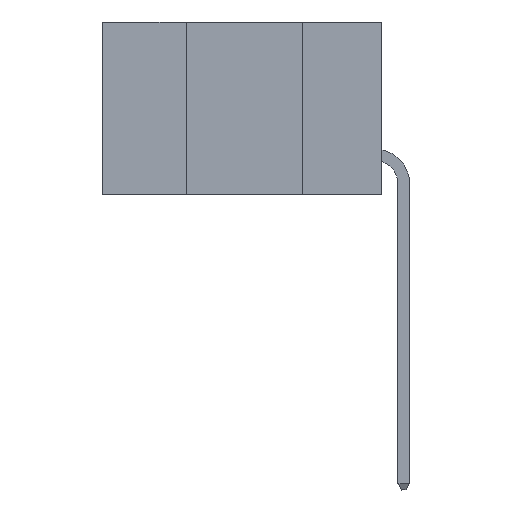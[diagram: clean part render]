
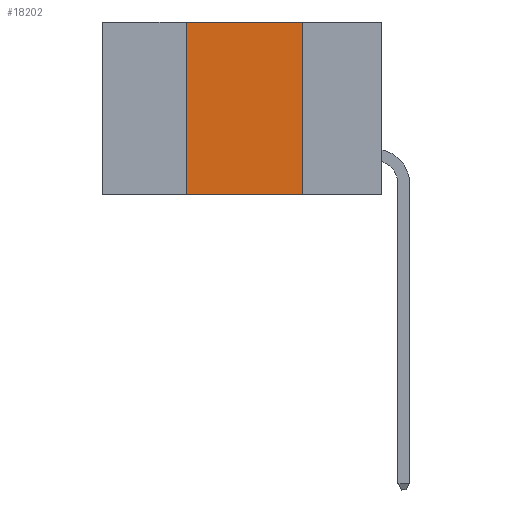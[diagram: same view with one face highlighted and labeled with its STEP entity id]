
A CAD part, left-side view. The second image highlights one B-rep face of the part: STEP entity #18202.
In plain terms, the highlighted planar face has unit normal (-1, 0, 0).
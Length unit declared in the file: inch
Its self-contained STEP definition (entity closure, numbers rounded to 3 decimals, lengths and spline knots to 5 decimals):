
#183 = CARTESIAN_POINT ( 'NONE',  ( 0., 0.17, 0. ) ) ;
#1536 = EDGE_CURVE ( 'NONE', #5941, #9464, #15123, .T. ) ;
#1832 = EDGE_LOOP ( 'NONE', ( #10894, #19282, #5438, #14898 ) ) ;
#2305 = CARTESIAN_POINT ( 'NONE',  ( 0., 0.42, 0. ) ) ;
#3840 = VECTOR ( 'NONE', #6556, 39.37008 ) ;
#4532 = PLANE ( 'NONE',  #10643 ) ;
#4639 = EDGE_CURVE ( 'NONE', #5941, #10305, #12330, .T. ) ;
#5438 = ORIENTED_EDGE ( 'NONE', *, *, #1536, .F. ) ;
#5863 = EDGE_CURVE ( 'NONE', #12023, #10305, #6042, .T. ) ;
#5941 = VERTEX_POINT ( 'NONE', #13922 ) ;
#5975 = LINE ( 'NONE', #20013, #3840 ) ;
#6042 = LINE ( 'NONE', #19173, #21668 ) ;
#6143 = DIRECTION ( 'NONE',  ( 0., 0., 1. ) ) ;
#6207 = DIRECTION ( 'NONE',  ( 1., 0., 0. ) ) ;
#6556 = DIRECTION ( 'NONE',  ( 0., -1., 0. ) ) ;
#8009 = CARTESIAN_POINT ( 'NONE',  ( 0., 0.6, 0. ) ) ;
#9464 = VERTEX_POINT ( 'NONE', #2305 ) ;
#10305 = VERTEX_POINT ( 'NONE', #13067 ) ;
#10643 = AXIS2_PLACEMENT_3D ( 'NONE', #8009, #6207, #11249 ) ;
#10894 = ORIENTED_EDGE ( 'NONE', *, *, #5863, .F. ) ;
#11249 = DIRECTION ( 'NONE',  ( 0., 0., -1. ) ) ;
#12023 = VERTEX_POINT ( 'NONE', #183 ) ;
#12330 = LINE ( 'NONE', #15758, #21082 ) ;
#13067 = CARTESIAN_POINT ( 'NONE',  ( 0., 0.17, -0.37 ) ) ;
#13922 = CARTESIAN_POINT ( 'NONE',  ( 0., 0.42, -0.37 ) ) ;
#14898 = ORIENTED_EDGE ( 'NONE', *, *, #4639, .T. ) ;
#14979 = EDGE_CURVE ( 'NONE', #9464, #12023, #5975, .T. ) ;
#15123 = LINE ( 'NONE', #17993, #18561 ) ;
#15758 = CARTESIAN_POINT ( 'NONE',  ( 0., 0.6, -0.37 ) ) ;
#16365 = FACE_OUTER_BOUND ( 'NONE', #1832, .T. ) ;
#17905 = DIRECTION ( 'NONE',  ( 0., -1., 0. ) ) ;
#17993 = CARTESIAN_POINT ( 'NONE',  ( 0., 0.42, 0. ) ) ;
#18202 = ADVANCED_FACE ( 'NONE', ( #16365 ), #4532, .F. ) ;
#18561 = VECTOR ( 'NONE', #6143, 39.37008 ) ;
#18887 = DIRECTION ( 'NONE',  ( 0., 0., -1. ) ) ;
#19173 = CARTESIAN_POINT ( 'NONE',  ( 0., 0.17, 0. ) ) ;
#19282 = ORIENTED_EDGE ( 'NONE', *, *, #14979, .F. ) ;
#20013 = CARTESIAN_POINT ( 'NONE',  ( 0., 0.6, 0. ) ) ;
#21082 = VECTOR ( 'NONE', #17905, 39.37008 ) ;
#21668 = VECTOR ( 'NONE', #18887, 39.37008 ) ;
